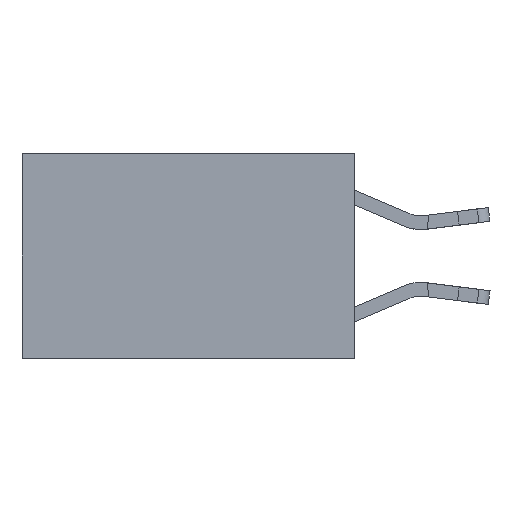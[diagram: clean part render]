
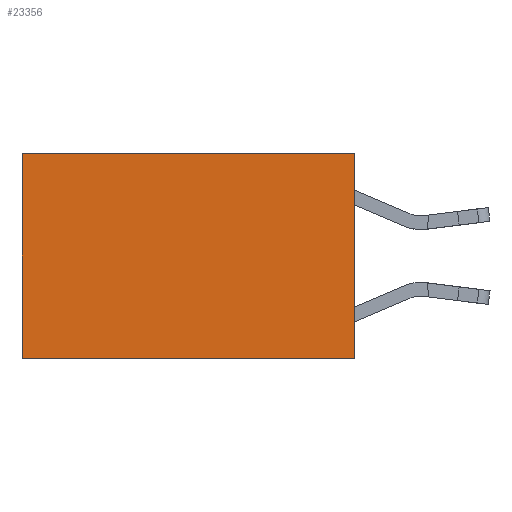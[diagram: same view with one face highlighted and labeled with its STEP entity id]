
A CAD part, left-side view. The second image highlights one B-rep face of the part: STEP entity #23356.
In plain terms, the highlighted planar face has unit normal (-1, 0, 0).
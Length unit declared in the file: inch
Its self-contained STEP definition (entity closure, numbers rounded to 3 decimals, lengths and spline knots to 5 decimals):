
#94 = VECTOR ( 'NONE', #17152, 39.37008 ) ;
#1482 = LINE ( 'NONE', #14899, #94 ) ;
#3119 = VERTEX_POINT ( 'NONE', #14471 ) ;
#3222 = PLANE ( 'NONE',  #17231 ) ;
#4100 = DIRECTION ( 'NONE',  ( 0., 0., -1. ) ) ;
#4309 = VECTOR ( 'NONE', #17037, 39.37008 ) ;
#5092 = VECTOR ( 'NONE', #10013, 39.37008 ) ;
#5161 = ORIENTED_EDGE ( 'NONE', *, *, #24086, .T. ) ;
#5508 = CARTESIAN_POINT ( 'NONE',  ( 0.2625, 0., 0. ) ) ;
#5514 = EDGE_CURVE ( 'NONE', #3119, #6410, #18489, .T. ) ;
#6410 = VERTEX_POINT ( 'NONE', #8301 ) ;
#6561 = VERTEX_POINT ( 'NONE', #16454 ) ;
#8301 = CARTESIAN_POINT ( 'NONE',  ( 0.2625, 0.6, -0.37 ) ) ;
#9739 = CARTESIAN_POINT ( 'NONE',  ( 0.2625, 0., 0. ) ) ;
#9971 = ORIENTED_EDGE ( 'NONE', *, *, #22913, .F. ) ;
#10013 = DIRECTION ( 'NONE',  ( 0., 1., 0. ) ) ;
#10577 = CARTESIAN_POINT ( 'NONE',  ( 0.2625, 0.6, 0. ) ) ;
#11981 = EDGE_LOOP ( 'NONE', ( #5161, #21127, #9971, #15360 ) ) ;
#12532 = LINE ( 'NONE', #10577, #4309 ) ;
#12645 = CARTESIAN_POINT ( 'NONE',  ( 0.2625, 0., 0. ) ) ;
#14471 = CARTESIAN_POINT ( 'NONE',  ( 0.2625, 0., -0.37 ) ) ;
#14899 = CARTESIAN_POINT ( 'NONE',  ( 0.2625, 0., 0. ) ) ;
#15360 = ORIENTED_EDGE ( 'NONE', *, *, #19240, .T. ) ;
#16454 = CARTESIAN_POINT ( 'NONE',  ( 0.2625, 0.6, 0. ) ) ;
#17037 = DIRECTION ( 'NONE',  ( 0., 0., -1. ) ) ;
#17152 = DIRECTION ( 'NONE',  ( 0., 1., 0. ) ) ;
#17231 = AXIS2_PLACEMENT_3D ( 'NONE', #9739, #27274, #25137 ) ;
#17702 = VERTEX_POINT ( 'NONE', #5508 ) ;
#18489 = LINE ( 'NONE', #24289, #5092 ) ;
#19240 = EDGE_CURVE ( 'NONE', #17702, #6561, #1482, .T. ) ;
#21127 = ORIENTED_EDGE ( 'NONE', *, *, #5514, .F. ) ;
#21189 = FACE_OUTER_BOUND ( 'NONE', #11981, .T. ) ;
#22913 = EDGE_CURVE ( 'NONE', #17702, #3119, #27100, .T. ) ;
#23356 = ADVANCED_FACE ( 'NONE', ( #21189 ), #3222, .F. ) ;
#24086 = EDGE_CURVE ( 'NONE', #6561, #6410, #12532, .T. ) ;
#24289 = CARTESIAN_POINT ( 'NONE',  ( 0.2625, 0., -0.37 ) ) ;
#25002 = VECTOR ( 'NONE', #4100, 39.37008 ) ;
#25137 = DIRECTION ( 'NONE',  ( 0., 0., -1. ) ) ;
#27100 = LINE ( 'NONE', #12645, #25002 ) ;
#27274 = DIRECTION ( 'NONE',  ( 1., 0., 0. ) ) ;
